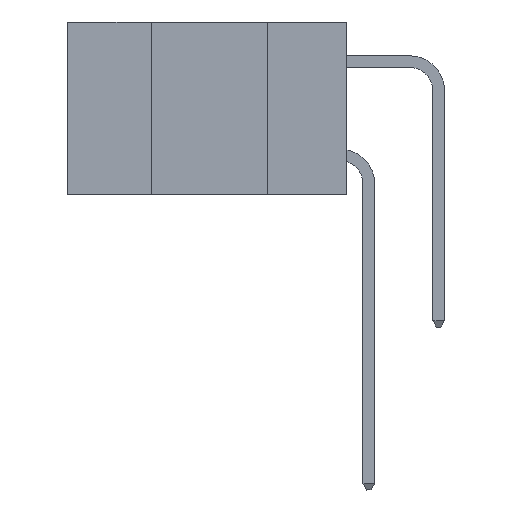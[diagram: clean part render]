
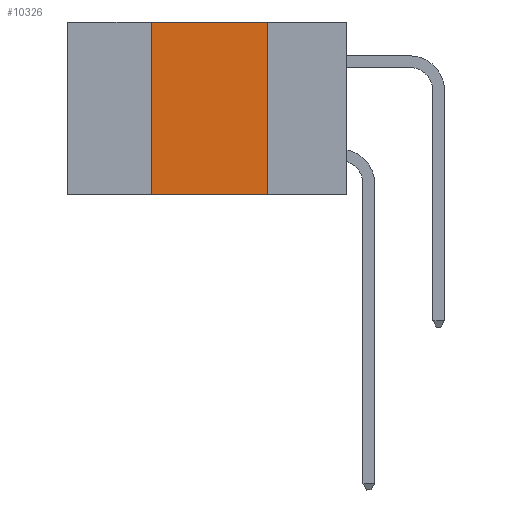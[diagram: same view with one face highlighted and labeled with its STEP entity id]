
A CAD part, left-side view. The second image highlights one B-rep face of the part: STEP entity #10326.
In plain terms, the highlighted planar face has unit normal (-1, 0, 0).
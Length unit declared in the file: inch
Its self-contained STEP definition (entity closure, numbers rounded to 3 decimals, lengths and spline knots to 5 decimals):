
#307 = DIRECTION ( 'NONE',  ( 0., -1., 0. ) ) ;
#425 = VECTOR ( 'NONE', #20173, 39.37008 ) ;
#916 = CARTESIAN_POINT ( 'NONE',  ( 0., 0.17, 0. ) ) ;
#1971 = LINE ( 'NONE', #11873, #26470 ) ;
#2389 = CARTESIAN_POINT ( 'NONE',  ( 0., 0.6, 0. ) ) ;
#3551 = CARTESIAN_POINT ( 'NONE',  ( 0., 0.42, 0. ) ) ;
#7490 = VERTEX_POINT ( 'NONE', #22437 ) ;
#7921 = CARTESIAN_POINT ( 'NONE',  ( 0., 0.17, 0. ) ) ;
#9724 = DIRECTION ( 'NONE',  ( 1., 0., 0. ) ) ;
#10326 = ADVANCED_FACE ( 'NONE', ( #26655 ), #11990, .F. ) ;
#10852 = ORIENTED_EDGE ( 'NONE', *, *, #20312, .T. ) ;
#10886 = EDGE_CURVE ( 'NONE', #12239, #28208, #25938, .T. ) ;
#11873 = CARTESIAN_POINT ( 'NONE',  ( 0., 0.6, -0.37 ) ) ;
#11990 = PLANE ( 'NONE',  #19312 ) ;
#12239 = VERTEX_POINT ( 'NONE', #916 ) ;
#16734 = DIRECTION ( 'NONE',  ( 0., 0., -1. ) ) ;
#16922 = ORIENTED_EDGE ( 'NONE', *, *, #25610, .F. ) ;
#18109 = VERTEX_POINT ( 'NONE', #27577 ) ;
#18257 = LINE ( 'NONE', #3551, #425 ) ;
#19210 = EDGE_LOOP ( 'NONE', ( #28352, #23789, #16922, #10852 ) ) ;
#19312 = AXIS2_PLACEMENT_3D ( 'NONE', #28559, #9724, #16734 ) ;
#20173 = DIRECTION ( 'NONE',  ( 0., 0., 1. ) ) ;
#20312 = EDGE_CURVE ( 'NONE', #18109, #28208, #1971, .T. ) ;
#21011 = CARTESIAN_POINT ( 'NONE',  ( 0., 0.17, -0.37 ) ) ;
#22437 = CARTESIAN_POINT ( 'NONE',  ( 0., 0.42, 0. ) ) ;
#23551 = DIRECTION ( 'NONE',  ( 0., -1., 0. ) ) ;
#23789 = ORIENTED_EDGE ( 'NONE', *, *, #29332, .F. ) ;
#24767 = DIRECTION ( 'NONE',  ( 0., 0., -1. ) ) ;
#25610 = EDGE_CURVE ( 'NONE', #18109, #7490, #18257, .T. ) ;
#25938 = LINE ( 'NONE', #7921, #29258 ) ;
#26197 = LINE ( 'NONE', #2389, #30288 ) ;
#26470 = VECTOR ( 'NONE', #307, 39.37008 ) ;
#26655 = FACE_OUTER_BOUND ( 'NONE', #19210, .T. ) ;
#27577 = CARTESIAN_POINT ( 'NONE',  ( 0., 0.42, -0.37 ) ) ;
#28208 = VERTEX_POINT ( 'NONE', #21011 ) ;
#28352 = ORIENTED_EDGE ( 'NONE', *, *, #10886, .F. ) ;
#28559 = CARTESIAN_POINT ( 'NONE',  ( 0., 0.6, 0. ) ) ;
#29258 = VECTOR ( 'NONE', #24767, 39.37008 ) ;
#29332 = EDGE_CURVE ( 'NONE', #7490, #12239, #26197, .T. ) ;
#30288 = VECTOR ( 'NONE', #23551, 39.37008 ) ;
